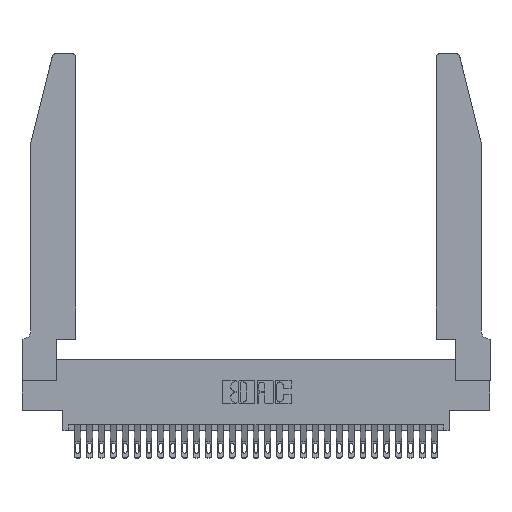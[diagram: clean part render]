
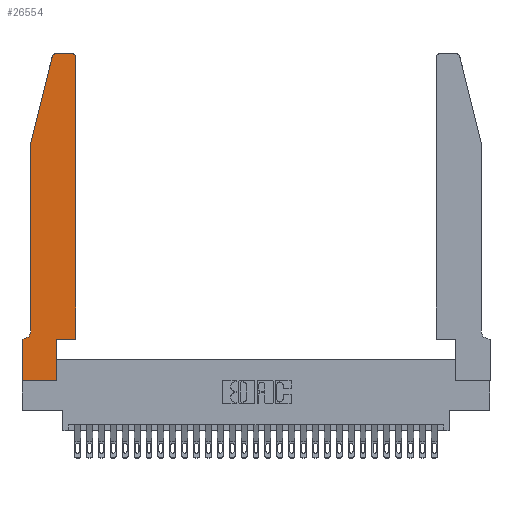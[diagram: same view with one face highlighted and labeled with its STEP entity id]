
A CAD part, top view. The second image highlights one B-rep face of the part: STEP entity #26554.
In plain terms, the highlighted planar face has unit normal (0, 0, 1).
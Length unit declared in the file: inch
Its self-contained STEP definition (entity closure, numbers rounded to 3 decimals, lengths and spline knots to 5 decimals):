
#370 = VERTEX_POINT ( 'NONE', #29494 ) ;
#653 = EDGE_CURVE ( 'NONE', #7698, #25915, #24167, .T. ) ;
#708 = VERTEX_POINT ( 'NONE', #23943 ) ;
#1062 = DIRECTION ( 'NONE',  ( 0., 1., 0. ) ) ;
#1326 = LINE ( 'NONE', #26134, #13525 ) ;
#1404 = DIRECTION ( 'NONE',  ( 1., 0., 0. ) ) ;
#1773 = DIRECTION ( 'NONE',  ( 0., -1., 0. ) ) ;
#2260 = AXIS2_PLACEMENT_3D ( 'NONE', #8619, #25207, #11069 ) ;
#2283 = CARTESIAN_POINT ( 'NONE',  ( 0.4505, 0.35, 0.37 ) ) ;
#2429 = CARTESIAN_POINT ( 'NONE',  ( 0.2605, 2.75, 0.37 ) ) ;
#3136 = ORIENTED_EDGE ( 'NONE', *, *, #11977, .T. ) ;
#3845 = CIRCLE ( 'NONE', #2260, 0.07 ) ;
#3855 = CARTESIAN_POINT ( 'NONE',  ( 0.0055, 0.35, 0.37 ) ) ;
#3937 = CARTESIAN_POINT ( 'NONE',  ( 0.2865, 0.35, 0.37 ) ) ;
#4211 = PLANE ( 'NONE',  #6217 ) ;
#4669 = CARTESIAN_POINT ( 'NONE',  ( 0., 0., 0.37 ) ) ;
#4798 = EDGE_CURVE ( 'NONE', #370, #9899, #1326, .T. ) ;
#5088 = VECTOR ( 'NONE', #24780, 39.37008 ) ;
#5118 = ORIENTED_EDGE ( 'NONE', *, *, #19953, .T. ) ;
#5406 = EDGE_CURVE ( 'NONE', #25915, #12038, #27920, .T. ) ;
#6036 = VECTOR ( 'NONE', #16467, 39.37008 ) ;
#6217 = AXIS2_PLACEMENT_3D ( 'NONE', #6690, #9210, #25779 ) ;
#6690 = CARTESIAN_POINT ( 'NONE',  ( 0., 0.35, 0.37 ) ) ;
#7698 = VERTEX_POINT ( 'NONE', #20546 ) ;
#7782 = VERTEX_POINT ( 'NONE', #27987 ) ;
#7980 = DIRECTION ( 'NONE',  ( -0.239, -0.971, 0. ) ) ;
#8619 = CARTESIAN_POINT ( 'NONE',  ( 0.0055, 0.42, 0.37 ) ) ;
#9032 = EDGE_CURVE ( 'NONE', #17659, #7698, #16654, .T. ) ;
#9210 = DIRECTION ( 'NONE',  ( 0., 0., 1. ) ) ;
#9556 = AXIS2_PLACEMENT_3D ( 'NONE', #30112, #15938, #1404 ) ;
#9745 = ORIENTED_EDGE ( 'NONE', *, *, #25458, .T. ) ;
#9899 = VERTEX_POINT ( 'NONE', #4669 ) ;
#10267 = FACE_OUTER_BOUND ( 'NONE', #23835, .T. ) ;
#10494 = ORIENTED_EDGE ( 'NONE', *, *, #5406, .T. ) ;
#11069 = DIRECTION ( 'NONE',  ( -1., 0., 0. ) ) ;
#11236 = CARTESIAN_POINT ( 'NONE',  ( 0.2865, 0., 0.37 ) ) ;
#11357 = VERTEX_POINT ( 'NONE', #11236 ) ;
#11495 = CARTESIAN_POINT ( 'NONE',  ( 0.4505, 0.35, 0.37 ) ) ;
#11949 = LINE ( 'NONE', #13249, #30807 ) ;
#11977 = EDGE_CURVE ( 'NONE', #12844, #17659, #22321, .T. ) ;
#12038 = VERTEX_POINT ( 'NONE', #24095 ) ;
#12367 = EDGE_CURVE ( 'NONE', #11357, #27739, #11949, .T. ) ;
#12374 = ORIENTED_EDGE ( 'NONE', *, *, #24266, .T. ) ;
#12389 = CARTESIAN_POINT ( 'NONE',  ( 0.284, 2.72, 0.37 ) ) ;
#12786 = CARTESIAN_POINT ( 'NONE',  ( 0.4505, 0.35, 0.37 ) ) ;
#12844 = VERTEX_POINT ( 'NONE', #12786 ) ;
#13249 = CARTESIAN_POINT ( 'NONE',  ( 0.2865, 0.35, 0.37 ) ) ;
#13513 = LINE ( 'NONE', #11495, #19081 ) ;
#13525 = VECTOR ( 'NONE', #30884, 39.37008 ) ;
#14061 = VECTOR ( 'NONE', #1773, 39.37008 ) ;
#14079 = CARTESIAN_POINT ( 'NONE',  ( 0.0755, 0.35, 0.37 ) ) ;
#14763 = DIRECTION ( 'NONE',  ( 1., 0., 0. ) ) ;
#14804 = LINE ( 'NONE', #16266, #14061 ) ;
#15079 = VERTEX_POINT ( 'NONE', #3855 ) ;
#15523 = LINE ( 'NONE', #19889, #27336 ) ;
#15938 = DIRECTION ( 'NONE',  ( 0., 0., 1. ) ) ;
#16049 = VECTOR ( 'NONE', #16780, 39.37008 ) ;
#16266 = CARTESIAN_POINT ( 'NONE',  ( 0.0755, 2., 0.37 ) ) ;
#16331 = EDGE_CURVE ( 'NONE', #708, #7782, #14804, .T. ) ;
#16467 = DIRECTION ( 'NONE',  ( -1., 0., 0. ) ) ;
#16647 = CARTESIAN_POINT ( 'NONE',  ( 0., 0., 0.37 ) ) ;
#16654 = CIRCLE ( 'NONE', #9556, 0.03 ) ;
#16780 = DIRECTION ( 'NONE',  ( 0., 1., 0. ) ) ;
#17659 = VERTEX_POINT ( 'NONE', #22692 ) ;
#18346 = EDGE_CURVE ( 'NONE', #15079, #370, #25076, .T. ) ;
#19081 = VECTOR ( 'NONE', #25643, 39.37008 ) ;
#19889 = CARTESIAN_POINT ( 'NONE',  ( 0.0755, 2., 0.37 ) ) ;
#19953 = EDGE_CURVE ( 'NONE', #27739, #12844, #13513, .T. ) ;
#20546 = CARTESIAN_POINT ( 'NONE',  ( 0.4205, 2.75, 0.37 ) ) ;
#20680 = ORIENTED_EDGE ( 'NONE', *, *, #22092, .T. ) ;
#20752 = ORIENTED_EDGE ( 'NONE', *, *, #16331, .T. ) ;
#21055 = CARTESIAN_POINT ( 'NONE',  ( 0.284, 2.75, 0.37 ) ) ;
#22092 = EDGE_CURVE ( 'NONE', #9899, #11357, #22612, .T. ) ;
#22321 = LINE ( 'NONE', #2283, #16049 ) ;
#22612 = LINE ( 'NONE', #16647, #24093 ) ;
#22692 = CARTESIAN_POINT ( 'NONE',  ( 0.4505, 2.72, 0.37 ) ) ;
#23835 = EDGE_LOOP ( 'NONE', ( #25393, #10494, #9745, #20752, #12374, #28264, #28516, #20680, #30304, #5118, #3136, #27302 ) ) ;
#23943 = CARTESIAN_POINT ( 'NONE',  ( 0.0755, 2., 0.37 ) ) ;
#23983 = AXIS2_PLACEMENT_3D ( 'NONE', #12389, #28935, #14763 ) ;
#24093 = VECTOR ( 'NONE', #30793, 39.37008 ) ;
#24095 = CARTESIAN_POINT ( 'NONE',  ( 0.25487, 2.72718, 0.37 ) ) ;
#24167 = LINE ( 'NONE', #2429, #5088 ) ;
#24266 = EDGE_CURVE ( 'NONE', #7782, #15079, #3845, .T. ) ;
#24780 = DIRECTION ( 'NONE',  ( -1., 0., 0. ) ) ;
#25076 = LINE ( 'NONE', #14079, #6036 ) ;
#25207 = DIRECTION ( 'NONE',  ( 0., 0., -1. ) ) ;
#25393 = ORIENTED_EDGE ( 'NONE', *, *, #653, .T. ) ;
#25458 = EDGE_CURVE ( 'NONE', #12038, #708, #15523, .T. ) ;
#25643 = DIRECTION ( 'NONE',  ( 1., 0., 0. ) ) ;
#25779 = DIRECTION ( 'NONE',  ( 1., 0., 0. ) ) ;
#25915 = VERTEX_POINT ( 'NONE', #21055 ) ;
#26134 = CARTESIAN_POINT ( 'NONE',  ( 0., 0., 0.37 ) ) ;
#26554 = ADVANCED_FACE ( 'NONE', ( #10267 ), #4211, .T. ) ;
#27302 = ORIENTED_EDGE ( 'NONE', *, *, #9032, .T. ) ;
#27336 = VECTOR ( 'NONE', #7980, 39.37008 ) ;
#27739 = VERTEX_POINT ( 'NONE', #3937 ) ;
#27920 = CIRCLE ( 'NONE', #23983, 0.03 ) ;
#27987 = CARTESIAN_POINT ( 'NONE',  ( 0.0755, 0.42, 0.37 ) ) ;
#28264 = ORIENTED_EDGE ( 'NONE', *, *, #18346, .T. ) ;
#28516 = ORIENTED_EDGE ( 'NONE', *, *, #4798, .T. ) ;
#28935 = DIRECTION ( 'NONE',  ( 0., 0., 1. ) ) ;
#29494 = CARTESIAN_POINT ( 'NONE',  ( 0., 0.35, 0.37 ) ) ;
#30112 = CARTESIAN_POINT ( 'NONE',  ( 0.4205, 2.72, 0.37 ) ) ;
#30304 = ORIENTED_EDGE ( 'NONE', *, *, #12367, .T. ) ;
#30793 = DIRECTION ( 'NONE',  ( 1., 0., 0. ) ) ;
#30807 = VECTOR ( 'NONE', #1062, 39.37008 ) ;
#30884 = DIRECTION ( 'NONE',  ( 0., -1., 0. ) ) ;
